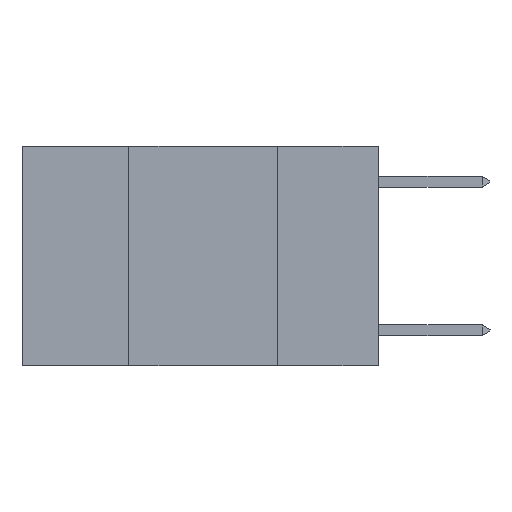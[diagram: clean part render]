
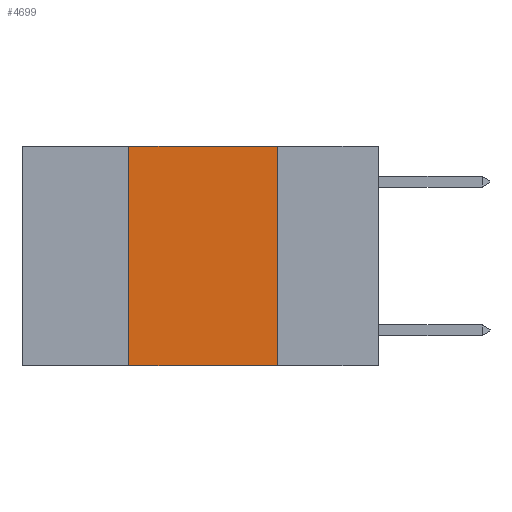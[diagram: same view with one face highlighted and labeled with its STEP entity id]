
A CAD part, left-side view. The second image highlights one B-rep face of the part: STEP entity #4699.
In plain terms, the highlighted planar face has unit normal (-1, 0, 0).
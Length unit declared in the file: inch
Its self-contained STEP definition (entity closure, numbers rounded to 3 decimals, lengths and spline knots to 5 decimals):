
#333 = CARTESIAN_POINT ( 'NONE',  ( 0., 0.42, 0. ) ) ;
#347 = DIRECTION ( 'NONE',  ( 0., -1., 0. ) ) ;
#584 = ORIENTED_EDGE ( 'NONE', *, *, #2455, .T. ) ;
#817 = AXIS2_PLACEMENT_3D ( 'NONE', #11098, #10678, #10631 ) ;
#852 = LINE ( 'NONE', #6829, #1147 ) ;
#1147 = VECTOR ( 'NONE', #6817, 39.37008 ) ;
#1574 = VERTEX_POINT ( 'NONE', #8397 ) ;
#2104 = DIRECTION ( 'NONE',  ( 0., 0., 1. ) ) ;
#2455 = EDGE_CURVE ( 'NONE', #1574, #8541, #4946, .T. ) ;
#2457 = EDGE_CURVE ( 'NONE', #1574, #6680, #7103, .T. ) ;
#2489 = EDGE_LOOP ( 'NONE', ( #10432, #6667, #2583, #584 ) ) ;
#2583 = ORIENTED_EDGE ( 'NONE', *, *, #2457, .F. ) ;
#3188 = VERTEX_POINT ( 'NONE', #6239 ) ;
#3999 = EDGE_CURVE ( 'NONE', #6680, #3188, #852, .T. ) ;
#4616 = CARTESIAN_POINT ( 'NONE',  ( 0., 0.17, -0.37 ) ) ;
#4626 = CARTESIAN_POINT ( 'NONE',  ( 0., 0.17, 0. ) ) ;
#4654 = VECTOR ( 'NONE', #347, 39.37008 ) ;
#4699 = ADVANCED_FACE ( 'NONE', ( #9736 ), #10720, .F. ) ;
#4911 = CARTESIAN_POINT ( 'NONE',  ( 0., 0.42, 0. ) ) ;
#4946 = LINE ( 'NONE', #9954, #4654 ) ;
#5553 = DIRECTION ( 'NONE',  ( 0., 0., -1. ) ) ;
#6239 = CARTESIAN_POINT ( 'NONE',  ( 0., 0.17, 0. ) ) ;
#6667 = ORIENTED_EDGE ( 'NONE', *, *, #3999, .F. ) ;
#6680 = VERTEX_POINT ( 'NONE', #4911 ) ;
#6817 = DIRECTION ( 'NONE',  ( 0., -1., 0. ) ) ;
#6829 = CARTESIAN_POINT ( 'NONE',  ( 0., 0.6, 0. ) ) ;
#7103 = LINE ( 'NONE', #333, #11579 ) ;
#7169 = EDGE_CURVE ( 'NONE', #3188, #8541, #9124, .T. ) ;
#8397 = CARTESIAN_POINT ( 'NONE',  ( 0., 0.42, -0.37 ) ) ;
#8541 = VERTEX_POINT ( 'NONE', #4616 ) ;
#9124 = LINE ( 'NONE', #4626, #11195 ) ;
#9736 = FACE_OUTER_BOUND ( 'NONE', #2489, .T. ) ;
#9954 = CARTESIAN_POINT ( 'NONE',  ( 0., 0.6, -0.37 ) ) ;
#10432 = ORIENTED_EDGE ( 'NONE', *, *, #7169, .F. ) ;
#10631 = DIRECTION ( 'NONE',  ( 0., 0., -1. ) ) ;
#10678 = DIRECTION ( 'NONE',  ( 1., 0., 0. ) ) ;
#10720 = PLANE ( 'NONE',  #817 ) ;
#11098 = CARTESIAN_POINT ( 'NONE',  ( 0., 0.6, 0. ) ) ;
#11195 = VECTOR ( 'NONE', #5553, 39.37008 ) ;
#11579 = VECTOR ( 'NONE', #2104, 39.37008 ) ;
